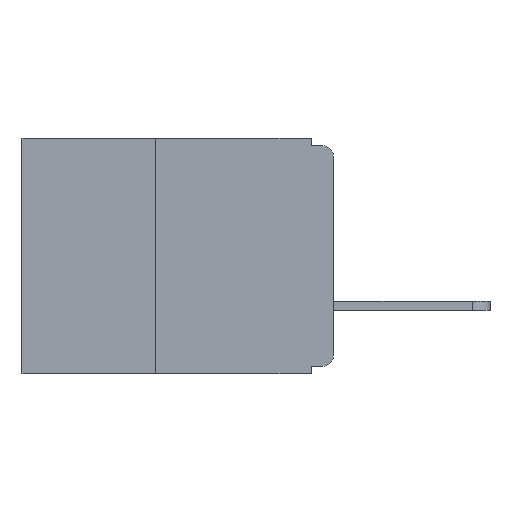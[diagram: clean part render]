
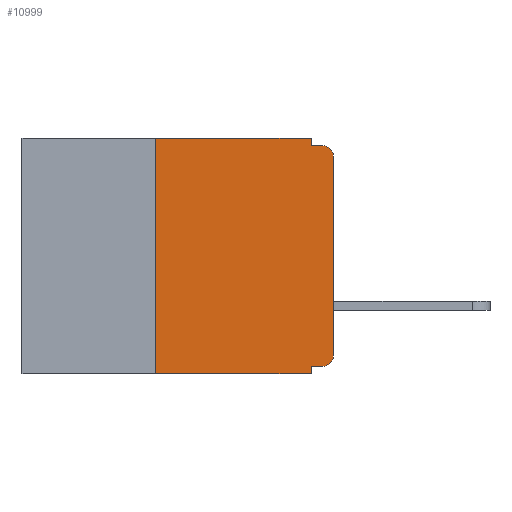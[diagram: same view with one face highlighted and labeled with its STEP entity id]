
A CAD part, left-side view. The second image highlights one B-rep face of the part: STEP entity #10999.
In plain terms, the highlighted planar face has unit normal (-1, 0, 0).
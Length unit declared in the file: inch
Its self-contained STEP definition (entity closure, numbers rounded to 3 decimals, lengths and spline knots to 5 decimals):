
#10 = EDGE_CURVE ( 'NONE', #7047, #11869, #24, .T. ) ;
#24 = LINE ( 'NONE', #19219, #85 ) ;
#85 = VECTOR ( 'NONE', #17413, 39.37008 ) ;
#223 = EDGE_CURVE ( 'NONE', #7047, #15254, #17149, .T. ) ;
#289 = EDGE_CURVE ( 'NONE', #3952, #15254, #16580, .T. ) ;
#562 = CARTESIAN_POINT ( 'NONE',  ( 0., 0.437, -0.33 ) ) ;
#839 = ORIENTED_EDGE ( 'NONE', *, *, #17360, .T. ) ;
#985 = VERTEX_POINT ( 'NONE', #6141 ) ;
#1075 = VERTEX_POINT ( 'NONE', #10324 ) ;
#1090 = ORIENTED_EDGE ( 'NONE', *, *, #4407, .T. ) ;
#1273 = EDGE_CURVE ( 'NONE', #15005, #985, #9835, .T. ) ;
#1358 = DIRECTION ( 'NONE',  ( 0., 0., 1. ) ) ;
#1583 = ORIENTED_EDGE ( 'NONE', *, *, #5963, .F. ) ;
#1741 = EDGE_CURVE ( 'NONE', #11869, #15005, #7641, .T. ) ;
#1810 = VECTOR ( 'NONE', #12793, 39.37008 ) ;
#1861 = ORIENTED_EDGE ( 'NONE', *, *, #1273, .F. ) ;
#1885 = LINE ( 'NONE', #12880, #1810 ) ;
#1930 = CARTESIAN_POINT ( 'NONE',  ( 0., 0., 0. ) ) ;
#2064 = ORIENTED_EDGE ( 'NONE', *, *, #1741, .F. ) ;
#2148 = ORIENTED_EDGE ( 'NONE', *, *, #10, .F. ) ;
#2514 = ORIENTED_EDGE ( 'NONE', *, *, #223, .T. ) ;
#2670 = ORIENTED_EDGE ( 'NONE', *, *, #289, .F. ) ;
#2689 = ORIENTED_EDGE ( 'NONE', *, *, #12781, .F. ) ;
#2836 = ORIENTED_EDGE ( 'NONE', *, *, #11604, .T. ) ;
#3155 = AXIS2_PLACEMENT_3D ( 'NONE', #18887, #18251, #18196 ) ;
#3454 = LINE ( 'NONE', #1930, #3494 ) ;
#3494 = VECTOR ( 'NONE', #1358, 39.37008 ) ;
#3952 = VERTEX_POINT ( 'NONE', #11558 ) ;
#4071 = DIRECTION ( 'NONE',  ( 0., 0., -1. ) ) ;
#4110 = DIRECTION ( 'NONE',  ( -1., 0., 0. ) ) ;
#4134 = CARTESIAN_POINT ( 'NONE',  ( 0., 0.015, -0.305 ) ) ;
#4137 = VECTOR ( 'NONE', #16958, 39.37008 ) ;
#4211 = LINE ( 'NONE', #18386, #4137 ) ;
#4407 = EDGE_CURVE ( 'NONE', #10333, #1075, #5719, .T. ) ;
#5701 = DIRECTION ( 'NONE',  ( 0., -1., 0. ) ) ;
#5719 = CIRCLE ( 'NONE', #6170, 0.015 ) ;
#5963 = EDGE_CURVE ( 'NONE', #985, #1075, #1885, .T. ) ;
#6141 = CARTESIAN_POINT ( 'NONE',  ( 0., 0.031, -0.01 ) ) ;
#6170 = AXIS2_PLACEMENT_3D ( 'NONE', #14960, #14903, #14868 ) ;
#6221 = DIRECTION ( 'NONE',  ( 0., 0., -1. ) ) ;
#7044 = AXIS2_PLACEMENT_3D ( 'NONE', #4134, #4110, #4071 ) ;
#7047 = VERTEX_POINT ( 'NONE', #16162 ) ;
#7359 = VECTOR ( 'NONE', #8498, 39.37008 ) ;
#7641 = LINE ( 'NONE', #10073, #7359 ) ;
#7657 = CARTESIAN_POINT ( 'NONE',  ( 0., 0.031, -0.33 ) ) ;
#7975 = CARTESIAN_POINT ( 'NONE',  ( 0., 0.031, -0.33 ) ) ;
#8235 = CARTESIAN_POINT ( 'NONE',  ( 0., 0.015, -0.32 ) ) ;
#8469 = CIRCLE ( 'NONE', #7044, 0.015 ) ;
#8498 = DIRECTION ( 'NONE',  ( 0., -1., 0. ) ) ;
#8563 = VERTEX_POINT ( 'NONE', #8235 ) ;
#9259 = VERTEX_POINT ( 'NONE', #9729 ) ;
#9459 = EDGE_LOOP ( 'NONE', ( #839, #1090, #1583, #1861, #2064, #2148, #2514, #2670, #2689, #2836 ) ) ;
#9646 = VECTOR ( 'NONE', #15671, 39.37008 ) ;
#9729 = CARTESIAN_POINT ( 'NONE',  ( 0., 0., -0.305 ) ) ;
#9835 = LINE ( 'NONE', #13168, #9646 ) ;
#10073 = CARTESIAN_POINT ( 'NONE',  ( 0., 0.437, 0. ) ) ;
#10324 = CARTESIAN_POINT ( 'NONE',  ( 0., 0.015, -0.01 ) ) ;
#10333 = VERTEX_POINT ( 'NONE', #11438 ) ;
#10999 = ADVANCED_FACE ( 'NONE', ( #11441 ), #18351, .F. ) ;
#11438 = CARTESIAN_POINT ( 'NONE',  ( 0., 0., -0.025 ) ) ;
#11441 = FACE_OUTER_BOUND ( 'NONE', #9459, .T. ) ;
#11486 = CARTESIAN_POINT ( 'NONE',  ( 0., 0.25, 0. ) ) ;
#11558 = CARTESIAN_POINT ( 'NONE',  ( 0., 0.031, -0.32 ) ) ;
#11604 = EDGE_CURVE ( 'NONE', #8563, #9259, #8469, .T. ) ;
#11869 = VERTEX_POINT ( 'NONE', #11486 ) ;
#12781 = EDGE_CURVE ( 'NONE', #8563, #3952, #4211, .T. ) ;
#12793 = DIRECTION ( 'NONE',  ( 0., -1., 0. ) ) ;
#12880 = CARTESIAN_POINT ( 'NONE',  ( 0., 0., -0.01 ) ) ;
#13168 = CARTESIAN_POINT ( 'NONE',  ( 0., 0.031, 0. ) ) ;
#14868 = DIRECTION ( 'NONE',  ( 0., 0., -1. ) ) ;
#14903 = DIRECTION ( 'NONE',  ( -1., 0., 0. ) ) ;
#14960 = CARTESIAN_POINT ( 'NONE',  ( 0., 0.015, -0.025 ) ) ;
#15005 = VERTEX_POINT ( 'NONE', #15928 ) ;
#15254 = VERTEX_POINT ( 'NONE', #7975 ) ;
#15671 = DIRECTION ( 'NONE',  ( 0., 0., -1. ) ) ;
#15928 = CARTESIAN_POINT ( 'NONE',  ( 0., 0.031, 0. ) ) ;
#16162 = CARTESIAN_POINT ( 'NONE',  ( 0., 0.25, -0.33 ) ) ;
#16413 = VECTOR ( 'NONE', #6221, 39.37008 ) ;
#16580 = LINE ( 'NONE', #7657, #16413 ) ;
#16958 = DIRECTION ( 'NONE',  ( 0., 1., 0. ) ) ;
#17098 = VECTOR ( 'NONE', #5701, 39.37008 ) ;
#17149 = LINE ( 'NONE', #562, #17098 ) ;
#17360 = EDGE_CURVE ( 'NONE', #9259, #10333, #3454, .T. ) ;
#17413 = DIRECTION ( 'NONE',  ( 0., 0., 1. ) ) ;
#18196 = DIRECTION ( 'NONE',  ( 0., 0., -1. ) ) ;
#18251 = DIRECTION ( 'NONE',  ( 1., 0., 0. ) ) ;
#18351 = PLANE ( 'NONE',  #3155 ) ;
#18386 = CARTESIAN_POINT ( 'NONE',  ( 0., 0., -0.32 ) ) ;
#18887 = CARTESIAN_POINT ( 'NONE',  ( 0., 0.437, 0. ) ) ;
#19219 = CARTESIAN_POINT ( 'NONE',  ( 0., 0.25, -0.33 ) ) ;
